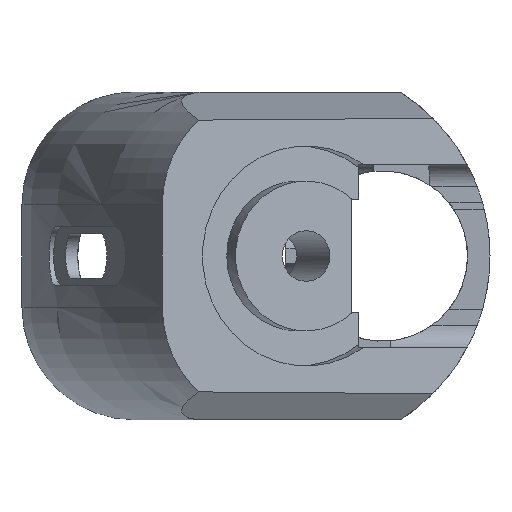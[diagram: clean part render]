
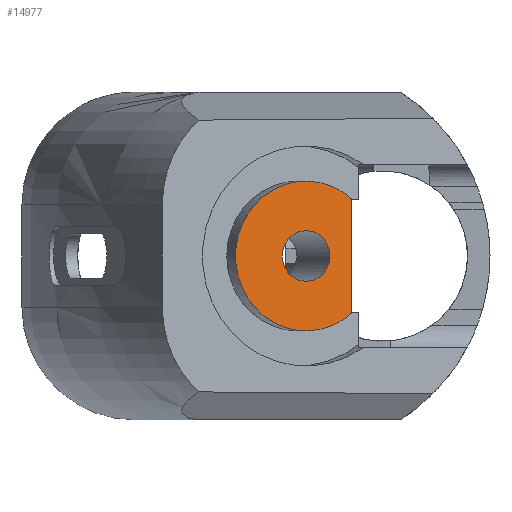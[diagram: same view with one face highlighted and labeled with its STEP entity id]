
A CAD part, left-side view. The second image highlights one B-rep face of the part: STEP entity #14977.
In plain terms, the highlighted planar face has unit normal (-0.943, -0.334, 0).
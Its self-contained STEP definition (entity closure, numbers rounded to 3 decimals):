
#3861 = PLANE('',#3862);
#3862 = AXIS2_PLACEMENT_3D('',#3863,#3864,#3865);
#3863 = CARTESIAN_POINT('',(-152.4,18.796,7.62));
#3864 = DIRECTION('',(0.,-1.,0.));
#3865 = DIRECTION('',(0.,0.,-1.));
#3915 = CYLINDRICAL_SURFACE('',#3916,3.429);
#3916 = AXIS2_PLACEMENT_3D('',#3917,#3918,#3919);
#3917 = CARTESIAN_POINT('',(-202.64,24.947,
    0.));
#3918 = DIRECTION('',(-0.943,-0.334,0.
    ));
#3919 = DIRECTION('',(0.334,-0.943,0.
    ));
#8735 = CYLINDRICAL_SURFACE('',#8736,10.16);
#8736 = AXIS2_PLACEMENT_3D('',#8737,#8738,#8739);
#8737 = CARTESIAN_POINT('',(-202.64,24.947,
    0.));
#8738 = DIRECTION('',(-0.943,-0.334,
    0.));
#8739 = DIRECTION('',(0.334,-0.943,0.)
  );
#8751 = VERTEX_POINT('',#8752);
#8752 = CARTESIAN_POINT('',(-200.461,18.796,7.62));
#8766 = PLANE('',#8767);
#8767 = AXIS2_PLACEMENT_3D('',#8768,#8769,#8770);
#8768 = CARTESIAN_POINT('',(-152.4,17.78,7.62));
#8769 = DIRECTION('',(0.,0.,-1.));
#8770 = DIRECTION('',(0.,1.,0.));
#8778 = EDGE_CURVE('',#8751,#8779,#8781,.T.);
#8779 = VERTEX_POINT('',#8780);
#8780 = CARTESIAN_POINT('',(-200.461,18.796,-7.62));
#8781 = SURFACE_CURVE('',#8782,(#8786,#8792),.PCURVE_S1.);
#8782 = LINE('',#8783,#8784);
#8783 = CARTESIAN_POINT('',(-200.461,18.796,-7.303));
#8784 = VECTOR('',#8785,1.);
#8785 = DIRECTION('',(0.,0.,-1.));
#8786 = PCURVE('',#3861,#8787);
#8787 = DEFINITIONAL_REPRESENTATION('',(#8788),#8791);
#8788 = B_SPLINE_CURVE_WITH_KNOTS('',1,(#8789,#8790),.UNSPECIFIED.,.F.,
  .F.,(2,2),(-14.923,0.318),.PIECEWISE_BEZIER_KNOTS.);
#8789 = CARTESIAN_POINT('',(0.,-48.061));
#8790 = CARTESIAN_POINT('',(15.24,-48.061));
#8791 = ( GEOMETRIC_REPRESENTATION_CONTEXT(2) 
PARAMETRIC_REPRESENTATION_CONTEXT() REPRESENTATION_CONTEXT('2D SPACE',''
  ) );
#8792 = PCURVE('',#8793,#8798);
#8793 = PLANE('',#8794);
#8794 = AXIS2_PLACEMENT_3D('',#8795,#8796,#8797);
#8795 = CARTESIAN_POINT('',(-209.55,44.45,-22.225));
#8796 = DIRECTION('',(0.943,0.334,0.));
#8797 = DIRECTION('',(0.334,-0.943,0.)
  );
#8798 = DEFINITIONAL_REPRESENTATION('',(#8799),#8802);
#8799 = B_SPLINE_CURVE_WITH_KNOTS('',1,(#8800,#8801),.UNSPECIFIED.,.F.,
  .F.,(2,2),(-14.923,0.318),.PIECEWISE_BEZIER_KNOTS.);
#8800 = CARTESIAN_POINT('',(27.216,-29.845));
#8801 = CARTESIAN_POINT('',(27.216,-14.605));
#8802 = ( GEOMETRIC_REPRESENTATION_CONTEXT(2) 
PARAMETRIC_REPRESENTATION_CONTEXT() REPRESENTATION_CONTEXT('2D SPACE',''
  ) );
#8820 = PLANE('',#8821);
#8821 = AXIS2_PLACEMENT_3D('',#8822,#8823,#8824);
#8822 = CARTESIAN_POINT('',(-152.4,18.796,-7.62));
#8823 = DIRECTION('',(0.,0.,1.));
#8824 = DIRECTION('',(0.,-1.,0.));
#8907 = EDGE_CURVE('',#8908,#8908,#8910,.T.);
#8908 = VERTEX_POINT('',#8909);
#8909 = CARTESIAN_POINT('',(-201.495,21.715,
    0.));
#8910 = SURFACE_CURVE('',#8911,(#8916,#8923),.PCURVE_S1.);
#8911 = CIRCLE('',#8912,3.429);
#8912 = AXIS2_PLACEMENT_3D('',#8913,#8914,#8915);
#8913 = CARTESIAN_POINT('',(-202.64,24.947,
    0.));
#8914 = DIRECTION('',(-0.943,-0.334,0.
    ));
#8915 = DIRECTION('',(0.334,-0.943,0.
    ));
#8916 = PCURVE('',#3915,#8917);
#8917 = DEFINITIONAL_REPRESENTATION('',(#8918),#8922);
#8918 = LINE('',#8919,#8920);
#8919 = CARTESIAN_POINT('',(0.,0.));
#8920 = VECTOR('',#8921,1.);
#8921 = DIRECTION('',(1.,0.));
#8922 = ( GEOMETRIC_REPRESENTATION_CONTEXT(2) 
PARAMETRIC_REPRESENTATION_CONTEXT() REPRESENTATION_CONTEXT('2D SPACE',''
  ) );
#8923 = PCURVE('',#8793,#8924);
#8924 = DEFINITIONAL_REPRESENTATION('',(#8925),#8933);
#8925 = ( BOUNDED_CURVE() B_SPLINE_CURVE(2,(#8926,#8927,#8928,#8929,
#8930,#8931,#8932),.UNSPECIFIED.,.T.,.F.) B_SPLINE_CURVE_WITH_KNOTS((1,2
    ,2,2,2,1),(-2.094,0.,2.094,4.189,
6.283,8.378),.UNSPECIFIED.) CURVE() 
GEOMETRIC_REPRESENTATION_ITEM() RATIONAL_B_SPLINE_CURVE((1.,0.5,1.,0.5,
1.,0.5,1.)) REPRESENTATION_ITEM('') );
#8926 = CARTESIAN_POINT('',(24.12,-22.225));
#8927 = CARTESIAN_POINT('',(24.12,-28.164));
#8928 = CARTESIAN_POINT('',(18.976,-25.195));
#8929 = CARTESIAN_POINT('',(13.833,-22.225));
#8930 = CARTESIAN_POINT('',(18.976,-19.255));
#8931 = CARTESIAN_POINT('',(24.12,-16.286));
#8932 = CARTESIAN_POINT('',(24.12,-22.225));
#8933 = ( GEOMETRIC_REPRESENTATION_CONTEXT(2) 
PARAMETRIC_REPRESENTATION_CONTEXT() REPRESENTATION_CONTEXT('2D SPACE',''
  ) );
#14883 = EDGE_CURVE('',#14884,#14886,#14888,.T.);
#14884 = VERTEX_POINT('',#14885);
#14885 = CARTESIAN_POINT('',(-200.396,18.613,
    7.62));
#14886 = VERTEX_POINT('',#14887);
#14887 = CARTESIAN_POINT('',(-200.396,18.613,-7.62));
#14888 = SURFACE_CURVE('',#14889,(#14894,#14901),.PCURVE_S1.);
#14889 = CIRCLE('',#14890,10.16);
#14890 = AXIS2_PLACEMENT_3D('',#14891,#14892,#14893);
#14891 = CARTESIAN_POINT('',(-202.64,24.947,
    0.));
#14892 = DIRECTION('',(-0.943,-0.334,
    0.));
#14893 = DIRECTION('',(0.334,-0.943,0.
    ));
#14894 = PCURVE('',#8735,#14895);
#14895 = DEFINITIONAL_REPRESENTATION('',(#14896),#14900);
#14896 = LINE('',#14897,#14898);
#14897 = CARTESIAN_POINT('',(0.,0.));
#14898 = VECTOR('',#14899,1.);
#14899 = DIRECTION('',(1.,0.));
#14900 = ( GEOMETRIC_REPRESENTATION_CONTEXT(2) 
PARAMETRIC_REPRESENTATION_CONTEXT() REPRESENTATION_CONTEXT('2D SPACE',''
  ) );
#14901 = PCURVE('',#8793,#14902);
#14902 = DEFINITIONAL_REPRESENTATION('',(#14903),#14911);
#14903 = ( BOUNDED_CURVE() B_SPLINE_CURVE(2,(#14904,#14905,#14906,#14907
    ,#14908,#14909,#14910),.UNSPECIFIED.,.T.,.F.) 
B_SPLINE_CURVE_WITH_KNOTS((1,2,2,2,2,1),(-2.094,0.,
    2.094,4.189,6.283,8.378),
.UNSPECIFIED.) CURVE() GEOMETRIC_REPRESENTATION_ITEM() 
RATIONAL_B_SPLINE_CURVE((1.,0.5,1.,0.5,1.,0.5,1.)) REPRESENTATION_ITEM(
  '') );
#14904 = CARTESIAN_POINT('',(30.851,-22.225));
#14905 = CARTESIAN_POINT('',(30.851,-39.823));
#14906 = CARTESIAN_POINT('',(15.611,-31.024));
#14907 = CARTESIAN_POINT('',(0.371,-22.225));
#14908 = CARTESIAN_POINT('',(15.611,-13.426));
#14909 = CARTESIAN_POINT('',(30.851,-4.627));
#14910 = CARTESIAN_POINT('',(30.851,-22.225));
#14911 = ( GEOMETRIC_REPRESENTATION_CONTEXT(2) 
PARAMETRIC_REPRESENTATION_CONTEXT() REPRESENTATION_CONTEXT('2D SPACE',''
  ) );
#14959 = EDGE_CURVE('',#8779,#14886,#14960,.T.);
#14960 = SURFACE_CURVE('',#14961,(#14965,#14971),.PCURVE_S1.);
#14961 = LINE('',#14962,#14963);
#14962 = CARTESIAN_POINT('',(-202.326,24.059,-7.62));
#14963 = VECTOR('',#14964,1.);
#14964 = DIRECTION('',(0.334,-0.943,0.
    ));
#14965 = PCURVE('',#8820,#14966);
#14966 = DEFINITIONAL_REPRESENTATION('',(#14967),#14970);
#14967 = B_SPLINE_CURVE_WITH_KNOTS('',1,(#14968,#14969),.UNSPECIFIED.,
  .F.,.F.,(2,2),(5.583,6.661),
  .PIECEWISE_BEZIER_KNOTS.);
#14968 = CARTESIAN_POINT('',(0.,-48.061));
#14969 = CARTESIAN_POINT('',(1.016,-47.701));
#14970 = ( GEOMETRIC_REPRESENTATION_CONTEXT(2) 
PARAMETRIC_REPRESENTATION_CONTEXT() REPRESENTATION_CONTEXT('2D SPACE',''
  ) );
#14971 = PCURVE('',#8793,#14972);
#14972 = DEFINITIONAL_REPRESENTATION('',(#14973),#14976);
#14973 = B_SPLINE_CURVE_WITH_KNOTS('',1,(#14974,#14975),.UNSPECIFIED.,
  .F.,.F.,(2,2),(5.583,6.661),
  .PIECEWISE_BEZIER_KNOTS.);
#14974 = CARTESIAN_POINT('',(27.216,-14.605));
#14975 = CARTESIAN_POINT('',(28.294,-14.605));
#14976 = ( GEOMETRIC_REPRESENTATION_CONTEXT(2) 
PARAMETRIC_REPRESENTATION_CONTEXT() REPRESENTATION_CONTEXT('2D SPACE',''
  ) );
#14977 = ADVANCED_FACE('',(#14978,#15002),#8793,.F.);
#14978 = FACE_BOUND('',#14979,.F.);
#14979 = EDGE_LOOP('',(#14980,#14981,#14982,#15001));
#14980 = ORIENTED_EDGE('',*,*,#14959,.T.);
#14981 = ORIENTED_EDGE('',*,*,#14883,.F.);
#14982 = ORIENTED_EDGE('',*,*,#14983,.T.);
#14983 = EDGE_CURVE('',#14884,#8751,#14984,.T.);
#14984 = SURFACE_CURVE('',#14985,(#14989,#14995),.PCURVE_S1.);
#14985 = LINE('',#14986,#14987);
#14986 = CARTESIAN_POINT('',(-202.166,23.607,7.62));
#14987 = VECTOR('',#14988,1.);
#14988 = DIRECTION('',(-0.334,0.943,
    0.));
#14989 = PCURVE('',#8793,#14990);
#14990 = DEFINITIONAL_REPRESENTATION('',(#14991),#14994);
#14991 = B_SPLINE_CURVE_WITH_KNOTS('',1,(#14992,#14993),.UNSPECIFIED.,
  .F.,.F.,(2,2),(-6.182,-5.104),
  .PIECEWISE_BEZIER_KNOTS.);
#14992 = CARTESIAN_POINT('',(28.294,-29.845));
#14993 = CARTESIAN_POINT('',(27.216,-29.845));
#14994 = ( GEOMETRIC_REPRESENTATION_CONTEXT(2) 
PARAMETRIC_REPRESENTATION_CONTEXT() REPRESENTATION_CONTEXT('2D SPACE',''
  ) );
#14995 = PCURVE('',#8766,#14996);
#14996 = DEFINITIONAL_REPRESENTATION('',(#14997),#15000);
#14997 = B_SPLINE_CURVE_WITH_KNOTS('',1,(#14998,#14999),.UNSPECIFIED.,
  .F.,.F.,(2,2),(-6.182,-5.104),
  .PIECEWISE_BEZIER_KNOTS.);
#14998 = CARTESIAN_POINT('',(0.,-47.701));
#14999 = CARTESIAN_POINT('',(1.016,-48.061));
#15000 = ( GEOMETRIC_REPRESENTATION_CONTEXT(2) 
PARAMETRIC_REPRESENTATION_CONTEXT() REPRESENTATION_CONTEXT('2D SPACE',''
  ) );
#15001 = ORIENTED_EDGE('',*,*,#8778,.T.);
#15002 = FACE_BOUND('',#15003,.F.);
#15003 = EDGE_LOOP('',(#15004));
#15004 = ORIENTED_EDGE('',*,*,#8907,.T.);
